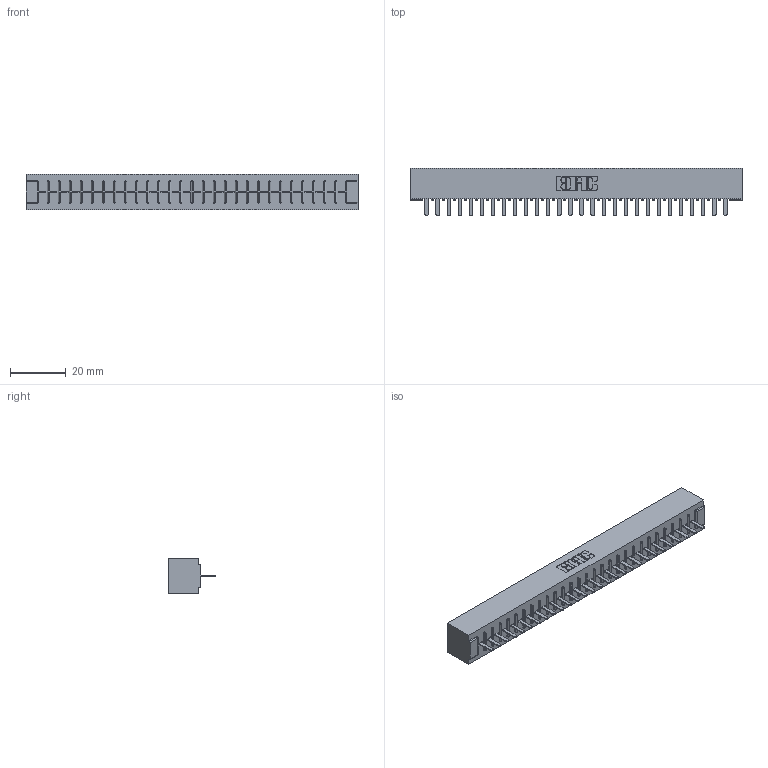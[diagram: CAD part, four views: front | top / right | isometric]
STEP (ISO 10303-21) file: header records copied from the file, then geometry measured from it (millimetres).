
FILE_DESCRIPTION (( 'STEP AP203' ), '1' );
FILE_NAME ('356-028-420-101.STEP', '2020-09-23T18:24:56', ( '' ), ( '' ), 'SwSTEP 2.0', 'SolidWorks 2020', '' );
FILE_SCHEMA (( 'CONFIG_CONTROL_DESIGN' ));
Length unit declared in the file: inch
Products named in the file (3): 306-290-001_120; 356-028-420-101; 306 Part_No Mounting
Assembly tree (29 placements, depth 2):
  356-028-420-101
    306 Part_No Mounting
    306-290-001_120  x28
Bounding box: 118.82 x 17.12 x 12.7 mm (x, y, z)
Volume: 13592.8 mm3; surface area: 13957.9 mm2
Topology: 29 solids, 29 shells, 2068 faces, 5808 edges, 3720 vertices
Faces by surface type: plane 1380, cylinder 576, sphere 112
Entity records: 27603 total; most frequent: CARTESIAN_POINT 4631, ORIENTED_EDGE 4588, DIRECTION 4568, EDGE_CURVE 2294, LINE 1790, VECTOR 1790, VERTEX_POINT 1452, AXIS2_PLACEMENT_3D 1389
